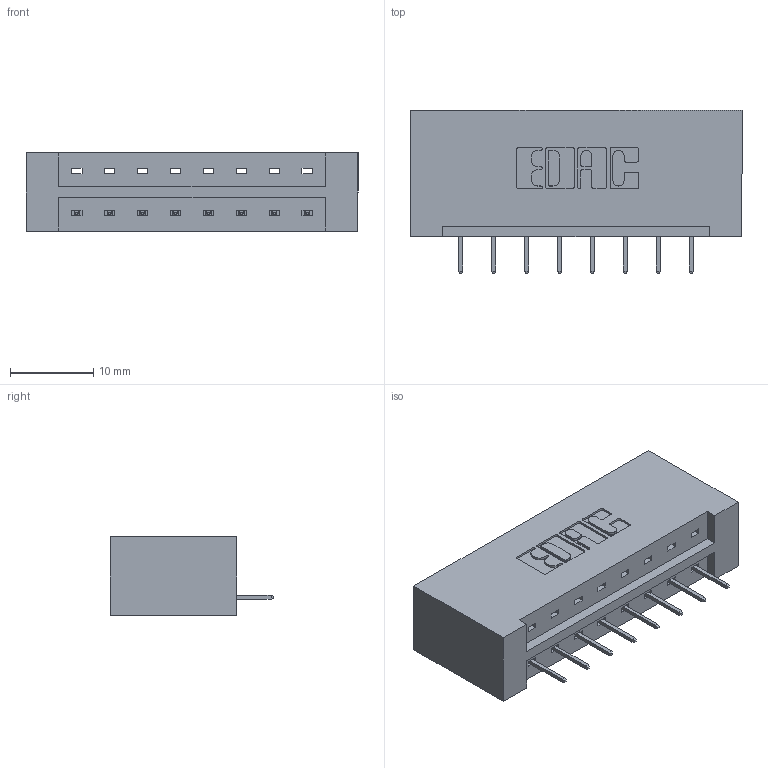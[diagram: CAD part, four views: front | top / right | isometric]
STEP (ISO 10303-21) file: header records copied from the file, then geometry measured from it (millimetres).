
FILE_DESCRIPTION (( 'STEP AP203' ), '1' );
FILE_NAME ('333-008-524-101.STEP', '2018-07-31T22:00:25', ( '' ), ( '' ), 'SwSTEP 2.0', 'SolidWorks 2016', '' );
FILE_SCHEMA (( 'CONFIG_CONTROL_DESIGN' ));
Length unit declared in the file: inch
Products named in the file (3): 345-292-001_345-293-124; 333-008-524-101; 333 Part_Lugless
Assembly tree (9 placements, depth 2):
  333-008-524-101
    333 Part_Lugless
    345-292-001_345-293-124  x8
Bounding box: 39.95 x 19.69 x 9.4 mm (x, y, z)
Volume: 4309.3 mm3; surface area: 4287.9 mm2
Topology: 9 solids, 9 shells, 602 faces, 1727 edges, 1118 vertices
Faces by surface type: plane 450, cylinder 152
Entity records: 9085 total; most frequent: CARTESIAN_POINT 1578, ORIENTED_EDGE 1522, DIRECTION 1393, EDGE_CURVE 761, VECTOR 645, LINE 645, VERTEX_POINT 502, AXIS2_PLACEMENT_3D 374
